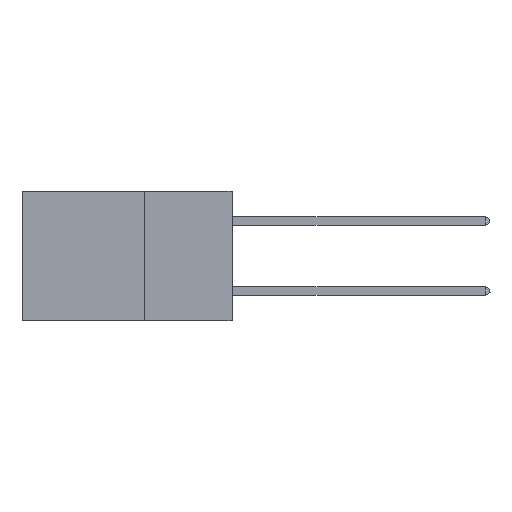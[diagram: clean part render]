
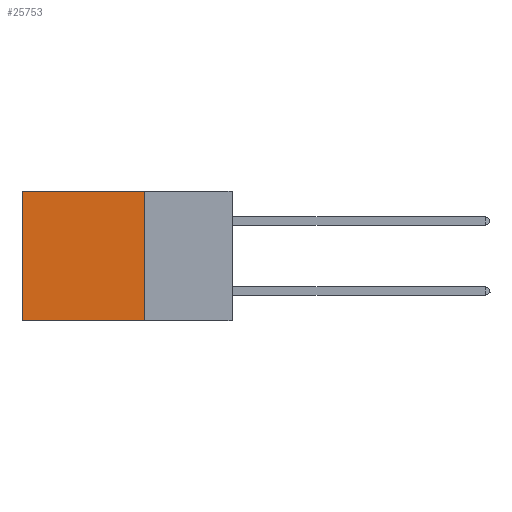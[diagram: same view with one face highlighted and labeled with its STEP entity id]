
A CAD part, left-side view. The second image highlights one B-rep face of the part: STEP entity #25753.
In plain terms, the highlighted planar face has unit normal (-1, 0, 0).
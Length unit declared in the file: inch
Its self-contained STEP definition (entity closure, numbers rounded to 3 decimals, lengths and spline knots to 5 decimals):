
#1071 = DIRECTION ( 'NONE',  ( 0., 1., 0. ) ) ;
#1178 = VECTOR ( 'NONE', #1071, 39.37008 ) ;
#2098 = DIRECTION ( 'NONE',  ( 0., 0., -1. ) ) ;
#2862 = DIRECTION ( 'NONE',  ( 1., 0., 0. ) ) ;
#3310 = EDGE_CURVE ( 'NONE', #27105, #31378, #14032, .T. ) ;
#4462 = AXIS2_PLACEMENT_3D ( 'NONE', #9974, #2862, #24985 ) ;
#5199 = CARTESIAN_POINT ( 'NONE',  ( 0.2875, 0.6, 0. ) ) ;
#5941 = LINE ( 'NONE', #18661, #33404 ) ;
#6461 = CARTESIAN_POINT ( 'NONE',  ( 0.2875, 0.25, -0.37 ) ) ;
#9516 = CARTESIAN_POINT ( 'NONE',  ( 0.2875, 0.25, -0.37 ) ) ;
#9974 = CARTESIAN_POINT ( 'NONE',  ( 0.2875, 0.25, 0. ) ) ;
#14032 = LINE ( 'NONE', #14240, #1178 ) ;
#14240 = CARTESIAN_POINT ( 'NONE',  ( 0.2875, 0.25, 0. ) ) ;
#16553 = VERTEX_POINT ( 'NONE', #9516 ) ;
#16811 = ORIENTED_EDGE ( 'NONE', *, *, #27945, .F. ) ;
#17109 = ORIENTED_EDGE ( 'NONE', *, *, #32761, .T. ) ;
#18368 = CARTESIAN_POINT ( 'NONE',  ( 0.2875, 0.25, 0. ) ) ;
#18661 = CARTESIAN_POINT ( 'NONE',  ( 0.2875, 0.6, 0. ) ) ;
#21881 = VECTOR ( 'NONE', #2098, 39.37008 ) ;
#22022 = CARTESIAN_POINT ( 'NONE',  ( 0.2875, 0.6, -0.37 ) ) ;
#22067 = PLANE ( 'NONE',  #4462 ) ;
#24985 = DIRECTION ( 'NONE',  ( 0., 0., -1. ) ) ;
#25753 = ADVANCED_FACE ( 'NONE', ( #40828 ), #22067, .F. ) ;
#26464 = VECTOR ( 'NONE', #41075, 39.37008 ) ;
#26969 = ORIENTED_EDGE ( 'NONE', *, *, #34925, .F. ) ;
#27105 = VERTEX_POINT ( 'NONE', #35420 ) ;
#27945 = EDGE_CURVE ( 'NONE', #16553, #39788, #31496, .T. ) ;
#27963 = LINE ( 'NONE', #18368, #21881 ) ;
#28653 = EDGE_LOOP ( 'NONE', ( #17109, #16811, #26969, #36455 ) ) ;
#31378 = VERTEX_POINT ( 'NONE', #5199 ) ;
#31384 = DIRECTION ( 'NONE',  ( 0., 0., -1. ) ) ;
#31496 = LINE ( 'NONE', #6461, #26464 ) ;
#32761 = EDGE_CURVE ( 'NONE', #31378, #39788, #5941, .T. ) ;
#33404 = VECTOR ( 'NONE', #31384, 39.37008 ) ;
#34925 = EDGE_CURVE ( 'NONE', #27105, #16553, #27963, .T. ) ;
#35420 = CARTESIAN_POINT ( 'NONE',  ( 0.2875, 0.25, 0. ) ) ;
#36455 = ORIENTED_EDGE ( 'NONE', *, *, #3310, .T. ) ;
#39788 = VERTEX_POINT ( 'NONE', #22022 ) ;
#40828 = FACE_OUTER_BOUND ( 'NONE', #28653, .T. ) ;
#41075 = DIRECTION ( 'NONE',  ( 0., 1., 0. ) ) ;
